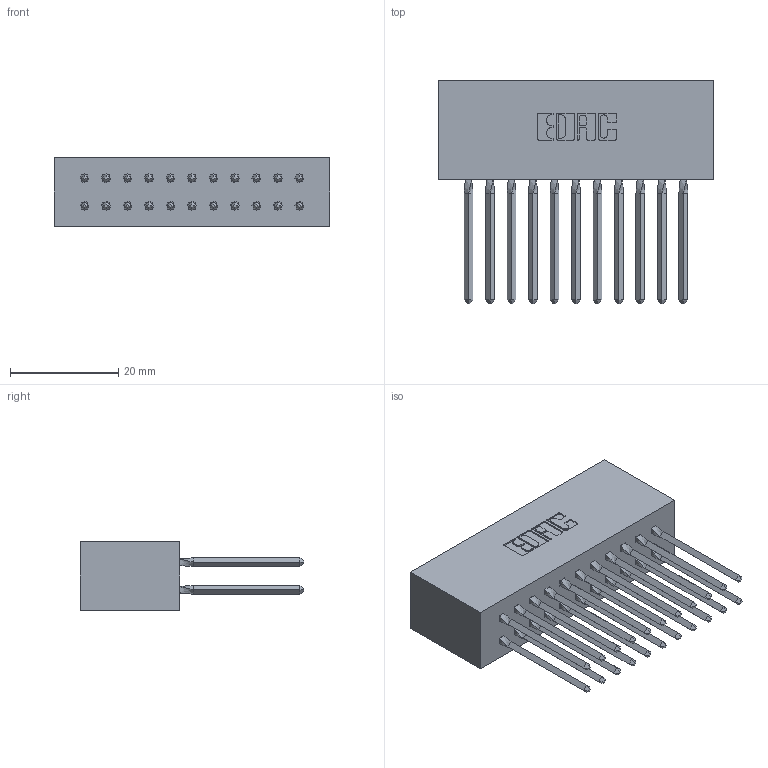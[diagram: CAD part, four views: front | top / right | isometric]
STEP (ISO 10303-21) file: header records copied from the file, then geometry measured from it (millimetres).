
FILE_DESCRIPTION (( 'STEP AP203' ), '1' );
FILE_NAME ('317-022-543-801.STEP', '2020-02-27T17:32:26', ( '' ), ( '' ), 'SwSTEP 2.0', 'SolidWorks 2016', '' );
FILE_SCHEMA (( 'CONFIG_CONTROL_DESIGN' ));
Length unit declared in the file: inch
Products named in the file (3): 317-022-543-801; 317-290-001_543; 317 Part_Lugless
Assembly tree (23 placements, depth 2):
  317-022-543-801
    317 Part_Lugless
    317-290-001_543  x22
Bounding box: 50.8 x 41.15 x 12.7 mm (x, y, z)
Volume: 9380.7 mm3; surface area: 13291.5 mm2
Topology: 23 solids, 23 shells, 2048 faces, 5673 edges, 3656 vertices
Faces by surface type: plane 1656, cylinder 304, bspline 88
Entity records: 19816 total; most frequent: CARTESIAN_POINT 3867, ORIENTED_EDGE 3366, DIRECTION 2805, EDGE_CURVE 1683, LINE 1435, VECTOR 1435, VERTEX_POINT 1115, AXIS2_PLACEMENT_3D 685
